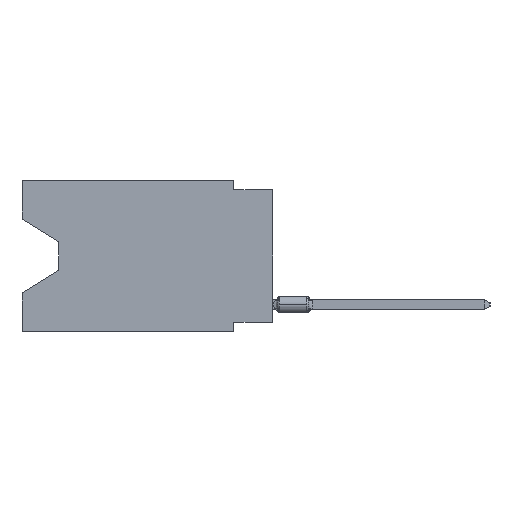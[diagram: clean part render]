
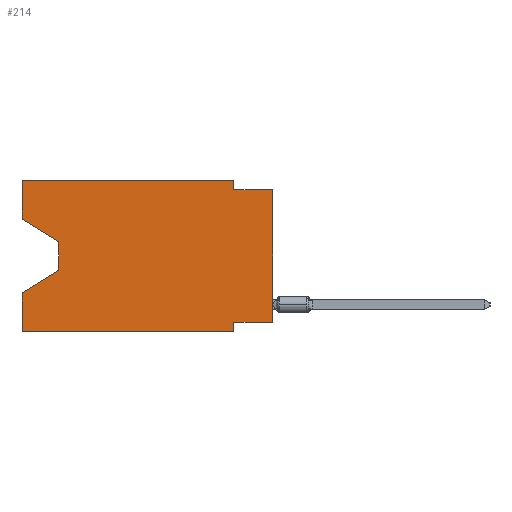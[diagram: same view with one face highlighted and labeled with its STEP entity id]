
A CAD part, left-side view. The second image highlights one B-rep face of the part: STEP entity #214.
In plain terms, the highlighted planar face has unit normal (-1, 0, 0).
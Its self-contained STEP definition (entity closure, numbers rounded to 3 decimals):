
#18 = LINE ( 'NONE', #41165, #58867 ) ;
#214 = ADVANCED_FACE ( 'NONE', ( #38665 ), #25732, .F. ) ;
#1066 = CARTESIAN_POINT ( 'NONE',  ( 0., 16.383, -7.36 ) ) ;
#1497 = LINE ( 'NONE', #15015, #36192 ) ;
#1831 = VECTOR ( 'NONE', #46976, 1000. ) ;
#2444 = VECTOR ( 'NONE', #17366, 1000. ) ;
#3366 = ORIENTED_EDGE ( 'NONE', *, *, #54444, .F. ) ;
#3547 = LINE ( 'NONE', #35980, #2444 ) ;
#3593 = ORIENTED_EDGE ( 'NONE', *, *, #29030, .F. ) ;
#4409 = VERTEX_POINT ( 'NONE', #36115 ) ;
#4753 = ORIENTED_EDGE ( 'NONE', *, *, #50312, .F. ) ;
#5119 = CARTESIAN_POINT ( 'NONE',  ( 0., 2.54, -9.906 ) ) ;
#5958 = VECTOR ( 'NONE', #15451, 1000. ) ;
#5982 = ORIENTED_EDGE ( 'NONE', *, *, #10574, .F. ) ;
#6307 = CARTESIAN_POINT ( 'NONE',  ( 0., 16.383, 0. ) ) ;
#6385 = ORIENTED_EDGE ( 'NONE', *, *, #16760, .T. ) ;
#7049 = VECTOR ( 'NONE', #12744, 1000. ) ;
#8374 = EDGE_CURVE ( 'NONE', #4409, #20940, #18, .T. ) ;
#9095 = CARTESIAN_POINT ( 'NONE',  ( 0., 16.383, -2.546 ) ) ;
#9131 = DIRECTION ( 'NONE',  ( 0., 0., 1. ) ) ;
#10409 = VECTOR ( 'NONE', #10554, 1000. ) ;
#10429 = LINE ( 'NONE', #38630, #26624 ) ;
#10554 = DIRECTION ( 'NONE',  ( 0., 0., 1. ) ) ;
#10574 = EDGE_CURVE ( 'NONE', #58935, #38764, #21281, .T. ) ;
#10762 = EDGE_CURVE ( 'NONE', #21188, #20940, #3547, .T. ) ;
#12252 = ORIENTED_EDGE ( 'NONE', *, *, #8374, .F. ) ;
#12744 = DIRECTION ( 'NONE',  ( 0., -1., 0. ) ) ;
#13487 = EDGE_CURVE ( 'NONE', #21188, #43191, #51688, .T. ) ;
#14504 = ORIENTED_EDGE ( 'NONE', *, *, #51580, .T. ) ;
#15015 = CARTESIAN_POINT ( 'NONE',  ( 0., 13.97, -4.013 ) ) ;
#15144 = CARTESIAN_POINT ( 'NONE',  ( 0., 0., 0. ) ) ;
#15234 = ORIENTED_EDGE ( 'NONE', *, *, #28581, .T. ) ;
#15446 = CARTESIAN_POINT ( 'NONE',  ( 0., 13.97, -5.893 ) ) ;
#15451 = DIRECTION ( 'NONE',  ( 0., -0.855, -0.519 ) ) ;
#15531 = DIRECTION ( 'NONE',  ( 0., 0., -1. ) ) ;
#15734 = LINE ( 'NONE', #15144, #1831 ) ;
#15745 = ORIENTED_EDGE ( 'NONE', *, *, #35912, .F. ) ;
#16424 = DIRECTION ( 'NONE',  ( 1., 0., 0. ) ) ;
#16760 = EDGE_CURVE ( 'NONE', #40909, #43191, #56570, .T. ) ;
#17366 = DIRECTION ( 'NONE',  ( 0., -1., 0. ) ) ;
#18151 = CARTESIAN_POINT ( 'NONE',  ( 0., 16.383, 0. ) ) ;
#18296 = EDGE_LOOP ( 'NONE', ( #14504, #15234, #6385, #42638, #43613, #12252, #3366, #41060, #15745, #3593, #5982, #4753 ) ) ;
#18899 = VERTEX_POINT ( 'NONE', #9095 ) ;
#19020 = VERTEX_POINT ( 'NONE', #51435 ) ;
#20934 = CARTESIAN_POINT ( 'NONE',  ( 0., 16.383, 0. ) ) ;
#20940 = VERTEX_POINT ( 'NONE', #5119 ) ;
#21188 = VERTEX_POINT ( 'NONE', #30886 ) ;
#21281 = LINE ( 'NONE', #6307, #38872 ) ;
#24045 = VERTEX_POINT ( 'NONE', #50584 ) ;
#24147 = CARTESIAN_POINT ( 'NONE',  ( 0., 16.383, 0. ) ) ;
#24505 = VERTEX_POINT ( 'NONE', #53404 ) ;
#25163 = CARTESIAN_POINT ( 'NONE',  ( 0., 13.97, -5.893 ) ) ;
#25732 = PLANE ( 'NONE',  #40107 ) ;
#26624 = VECTOR ( 'NONE', #15531, 1000. ) ;
#28581 = EDGE_CURVE ( 'NONE', #24045, #40909, #1497, .T. ) ;
#28823 = CARTESIAN_POINT ( 'NONE',  ( 0., 0., -9.271 ) ) ;
#28966 = CARTESIAN_POINT ( 'NONE',  ( 0., 16.383, -2.546 ) ) ;
#29030 = EDGE_CURVE ( 'NONE', #38764, #19020, #10429, .T. ) ;
#30184 = VECTOR ( 'NONE', #38120, 1000. ) ;
#30491 = EDGE_CURVE ( 'NONE', #55664, #24505, #15734, .T. ) ;
#30886 = CARTESIAN_POINT ( 'NONE',  ( 0., 16.383, -9.906 ) ) ;
#31611 = VECTOR ( 'NONE', #43633, 1000. ) ;
#33958 = CARTESIAN_POINT ( 'NONE',  ( 0., 16.383, 0. ) ) ;
#34212 = DIRECTION ( 'NONE',  ( 0., -1., 0. ) ) ;
#35912 = EDGE_CURVE ( 'NONE', #19020, #24505, #53296, .T. ) ;
#35980 = CARTESIAN_POINT ( 'NONE',  ( 0., 16.383, -9.906 ) ) ;
#36115 = CARTESIAN_POINT ( 'NONE',  ( 0., 2.54, -9.271 ) ) ;
#36192 = VECTOR ( 'NONE', #42921, 1000. ) ;
#38120 = DIRECTION ( 'NONE',  ( 0., 1., 0. ) ) ;
#38630 = CARTESIAN_POINT ( 'NONE',  ( 0., 2.54, 0. ) ) ;
#38665 = FACE_OUTER_BOUND ( 'NONE', #18296, .T. ) ;
#38764 = VERTEX_POINT ( 'NONE', #40811 ) ;
#38872 = VECTOR ( 'NONE', #34212, 1000. ) ;
#40107 = AXIS2_PLACEMENT_3D ( 'NONE', #20934, #16424, #57258 ) ;
#40811 = CARTESIAN_POINT ( 'NONE',  ( 0., 2.54, 0. ) ) ;
#40909 = VERTEX_POINT ( 'NONE', #25163 ) ;
#41060 = ORIENTED_EDGE ( 'NONE', *, *, #30491, .T. ) ;
#41165 = CARTESIAN_POINT ( 'NONE',  ( 0., 2.54, -9.906 ) ) ;
#42334 = LINE ( 'NONE', #28823, #30184 ) ;
#42638 = ORIENTED_EDGE ( 'NONE', *, *, #13487, .F. ) ;
#42921 = DIRECTION ( 'NONE',  ( 0., 0., -1. ) ) ;
#43191 = VERTEX_POINT ( 'NONE', #1066 ) ;
#43613 = ORIENTED_EDGE ( 'NONE', *, *, #10762, .T. ) ;
#43633 = DIRECTION ( 'NONE',  ( 0., 0.855, -0.519 ) ) ;
#45170 = CARTESIAN_POINT ( 'NONE',  ( 0., 0., -0.635 ) ) ;
#46976 = DIRECTION ( 'NONE',  ( 0., 0., 1. ) ) ;
#48005 = VECTOR ( 'NONE', #9131, 1000. ) ;
#50312 = EDGE_CURVE ( 'NONE', #18899, #58935, #59265, .T. ) ;
#50584 = CARTESIAN_POINT ( 'NONE',  ( 0., 13.97, -4.013 ) ) ;
#51372 = CARTESIAN_POINT ( 'NONE',  ( 0., 0., -9.271 ) ) ;
#51435 = CARTESIAN_POINT ( 'NONE',  ( 0., 2.54, -0.635 ) ) ;
#51580 = EDGE_CURVE ( 'NONE', #18899, #24045, #52657, .T. ) ;
#51688 = LINE ( 'NONE', #33958, #10409 ) ;
#52657 = LINE ( 'NONE', #28966, #5958 ) ;
#53296 = LINE ( 'NONE', #45170, #7049 ) ;
#53404 = CARTESIAN_POINT ( 'NONE',  ( 0., 0., -0.635 ) ) ;
#54444 = EDGE_CURVE ( 'NONE', #55664, #4409, #42334, .T. ) ;
#55664 = VERTEX_POINT ( 'NONE', #51372 ) ;
#56570 = LINE ( 'NONE', #15446, #31611 ) ;
#57258 = DIRECTION ( 'NONE',  ( 0., 0., -1. ) ) ;
#58867 = VECTOR ( 'NONE', #59169, 1000. ) ;
#58935 = VERTEX_POINT ( 'NONE', #24147 ) ;
#59169 = DIRECTION ( 'NONE',  ( 0., 0., -1. ) ) ;
#59265 = LINE ( 'NONE', #18151, #48005 ) ;
